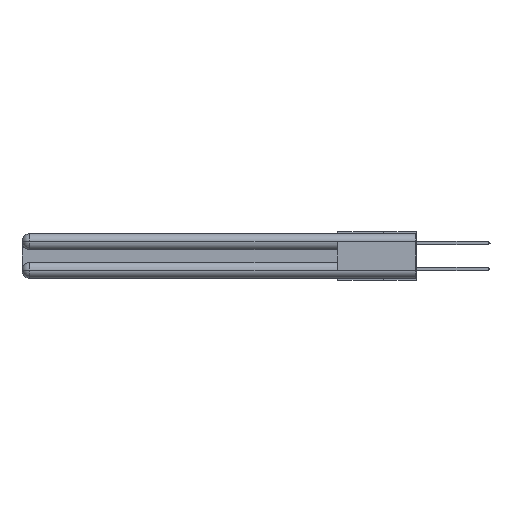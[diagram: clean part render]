
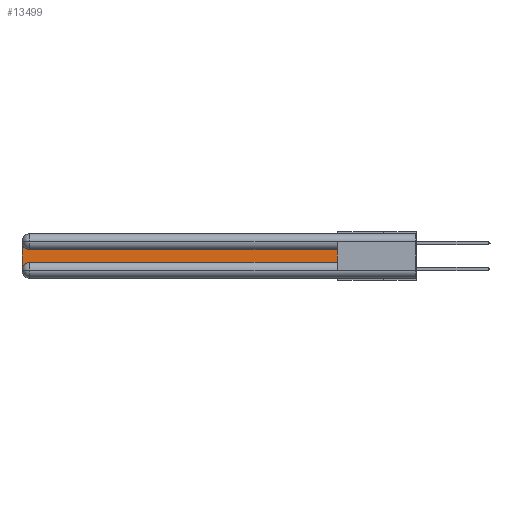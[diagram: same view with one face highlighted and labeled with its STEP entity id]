
A CAD part, left-side view. The second image highlights one B-rep face of the part: STEP entity #13499.
In plain terms, the highlighted planar face has unit normal (-1, 0, 0).
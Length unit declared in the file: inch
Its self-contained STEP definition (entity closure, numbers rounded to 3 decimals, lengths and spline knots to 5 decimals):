
#1747 = DIRECTION ( 'NONE',  ( 0., 0., -1. ) ) ;
#1824 = EDGE_CURVE ( 'NONE', #22979, #20480, #8950, .T. ) ;
#2376 = ORIENTED_EDGE ( 'NONE', *, *, #24479, .T. ) ;
#3214 = EDGE_CURVE ( 'NONE', #27461, #22979, #12645, .T. ) ;
#3709 = DIRECTION ( 'NONE',  ( 1., 0., 0. ) ) ;
#4224 = CARTESIAN_POINT ( 'NONE',  ( 0.075, 0.6, -0.2175 ) ) ;
#4890 = LINE ( 'NONE', #6488, #10021 ) ;
#5369 = VERTEX_POINT ( 'NONE', #7521 ) ;
#5434 = ORIENTED_EDGE ( 'NONE', *, *, #12308, .T. ) ;
#6043 = VECTOR ( 'NONE', #19041, 39.37008 ) ;
#6488 = CARTESIAN_POINT ( 'NONE',  ( 0.075, 0.6, -0.1225 ) ) ;
#7521 = CARTESIAN_POINT ( 'NONE',  ( 0.075, 0.6, -0.2175 ) ) ;
#8950 = LINE ( 'NONE', #18698, #23205 ) ;
#9461 = VECTOR ( 'NONE', #13277, 39.37008 ) ;
#9929 = CARTESIAN_POINT ( 'NONE',  ( 0.075, 3., -0.0625 ) ) ;
#10021 = VECTOR ( 'NONE', #15219, 39.37008 ) ;
#10825 = CARTESIAN_POINT ( 'NONE',  ( 0.075, 2.94, -0.0625 ) ) ;
#12308 = EDGE_CURVE ( 'NONE', #13777, #5369, #13224, .T. ) ;
#12510 = LINE ( 'NONE', #21199, #9461 ) ;
#12645 = CIRCLE ( 'NONE', #15030, 0.06 ) ;
#12715 = CARTESIAN_POINT ( 'NONE',  ( 0.075, 0.6, -0.1225 ) ) ;
#12805 = CIRCLE ( 'NONE', #21087, 0.06 ) ;
#12890 = VERTEX_POINT ( 'NONE', #12715 ) ;
#13224 = LINE ( 'NONE', #4224, #6043 ) ;
#13277 = DIRECTION ( 'NONE',  ( 0., 0., 1. ) ) ;
#13310 = DIRECTION ( 'NONE',  ( 1., 0., 0. ) ) ;
#13499 = ADVANCED_FACE ( 'NONE', ( #14794 ), #19105, .F. ) ;
#13777 = VERTEX_POINT ( 'NONE', #27332 ) ;
#13977 = ORIENTED_EDGE ( 'NONE', *, *, #17839, .T. ) ;
#14627 = CARTESIAN_POINT ( 'NONE',  ( 0.075, 2.94, -0.2775 ) ) ;
#14794 = FACE_OUTER_BOUND ( 'NONE', #16243, .T. ) ;
#15030 = AXIS2_PLACEMENT_3D ( 'NONE', #10825, #13310, #19334 ) ;
#15219 = DIRECTION ( 'NONE',  ( 0., 1., 0. ) ) ;
#16243 = EDGE_LOOP ( 'NONE', ( #13977, #23622, #19730, #2376, #5434, #20686 ) ) ;
#16900 = DIRECTION ( 'NONE',  ( 0., 0., -1. ) ) ;
#17839 = EDGE_CURVE ( 'NONE', #12890, #27461, #4890, .T. ) ;
#18432 = DIRECTION ( 'NONE',  ( 0., 0., -1. ) ) ;
#18698 = CARTESIAN_POINT ( 'NONE',  ( 0.075, 3., -0.2175 ) ) ;
#19041 = DIRECTION ( 'NONE',  ( 0., -1., 0. ) ) ;
#19105 = PLANE ( 'NONE',  #27152 ) ;
#19334 = DIRECTION ( 'NONE',  ( 0., 0., -1. ) ) ;
#19730 = ORIENTED_EDGE ( 'NONE', *, *, #1824, .T. ) ;
#20480 = VERTEX_POINT ( 'NONE', #27276 ) ;
#20686 = ORIENTED_EDGE ( 'NONE', *, *, #24035, .T. ) ;
#21087 = AXIS2_PLACEMENT_3D ( 'NONE', #14627, #3709, #16900 ) ;
#21199 = CARTESIAN_POINT ( 'NONE',  ( 0.075, 0.6, -0.2175 ) ) ;
#22979 = VERTEX_POINT ( 'NONE', #9929 ) ;
#23205 = VECTOR ( 'NONE', #18432, 39.37008 ) ;
#23622 = ORIENTED_EDGE ( 'NONE', *, *, #3214, .T. ) ;
#23654 = CARTESIAN_POINT ( 'NONE',  ( 0.075, 2.94, -0.1225 ) ) ;
#24035 = EDGE_CURVE ( 'NONE', #5369, #12890, #12510, .T. ) ;
#24479 = EDGE_CURVE ( 'NONE', #20480, #13777, #12805, .T. ) ;
#25547 = DIRECTION ( 'NONE',  ( 1., 0., 0. ) ) ;
#27152 = AXIS2_PLACEMENT_3D ( 'NONE', #27748, #25547, #1747 ) ;
#27276 = CARTESIAN_POINT ( 'NONE',  ( 0.075, 3., -0.2775 ) ) ;
#27332 = CARTESIAN_POINT ( 'NONE',  ( 0.075, 2.94, -0.2175 ) ) ;
#27461 = VERTEX_POINT ( 'NONE', #23654 ) ;
#27748 = CARTESIAN_POINT ( 'NONE',  ( 0.075, 3., -0.1225 ) ) ;
